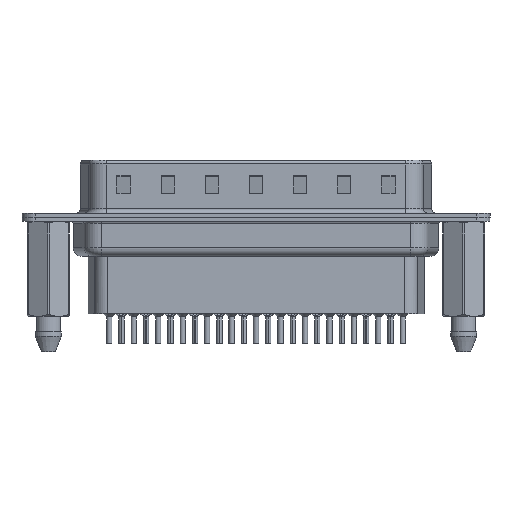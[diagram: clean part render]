
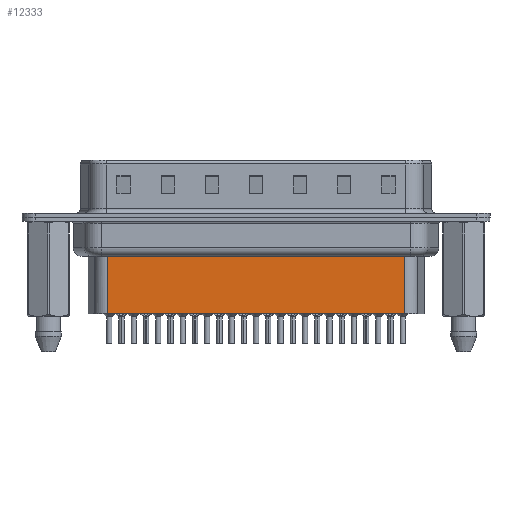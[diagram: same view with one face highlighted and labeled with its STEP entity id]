
A CAD part, front view. The second image highlights one B-rep face of the part: STEP entity #12333.
In plain terms, the highlighted planar face has unit normal (0, -1, 0).
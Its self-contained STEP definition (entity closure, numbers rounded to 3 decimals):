
#512 = VECTOR ( 'NONE', #2384, 1000. ) ;
#756 = CARTESIAN_POINT ( 'NONE',  ( 6.706, -3.5, -3.1 ) ) ;
#787 = FACE_OUTER_BOUND ( 'NONE', #13204, .T. ) ;
#915 = VECTOR ( 'NONE', #7128, 1000. ) ;
#1347 = DIRECTION ( 'NONE',  ( -1., 0., 0. ) ) ;
#1671 = AXIS2_PLACEMENT_3D ( 'NONE', #18731, #20494, #11427 ) ;
#1824 = VERTEX_POINT ( 'NONE', #12395 ) ;
#2384 = DIRECTION ( 'NONE',  ( 0., 0., -1. ) ) ;
#2472 = VERTEX_POINT ( 'NONE', #3318 ) ;
#3318 = CARTESIAN_POINT ( 'NONE',  ( 40.344, -3.5, -10.95 ) ) ;
#4831 = ORIENTED_EDGE ( 'NONE', *, *, #15955, .F. ) ;
#6227 = EDGE_CURVE ( 'NONE', #1824, #2472, #9227, .T. ) ;
#7128 = DIRECTION ( 'NONE',  ( -1., 0., 0. ) ) ;
#7300 = LINE ( 'NONE', #756, #17808 ) ;
#7325 = CARTESIAN_POINT ( 'NONE',  ( 6.706, -3.5, -10.95 ) ) ;
#9227 = LINE ( 'NONE', #20059, #512 ) ;
#9673 = PLANE ( 'NONE',  #1671 ) ;
#11427 = DIRECTION ( 'NONE',  ( 1., 0., 0. ) ) ;
#12333 = ADVANCED_FACE ( 'NONE', ( #787 ), #9673, .T. ) ;
#12395 = CARTESIAN_POINT ( 'NONE',  ( 40.344, -3.5, -4.097 ) ) ;
#12440 = LINE ( 'NONE', #21344, #27753 ) ;
#13204 = EDGE_LOOP ( 'NONE', ( #22185, #24298, #17603, #4831 ) ) ;
#13380 = CARTESIAN_POINT ( 'NONE',  ( 6.706, -3.5, -4.097 ) ) ;
#15955 = EDGE_CURVE ( 'NONE', #2472, #22702, #12440, .T. ) ;
#17603 = ORIENTED_EDGE ( 'NONE', *, *, #24813, .T. ) ;
#17808 = VECTOR ( 'NONE', #25112, 1000. ) ;
#18731 = CARTESIAN_POINT ( 'NONE',  ( 6.706, -3.5, -3.1 ) ) ;
#20059 = CARTESIAN_POINT ( 'NONE',  ( 40.344, -3.5, -3.1 ) ) ;
#20494 = DIRECTION ( 'NONE',  ( 0., -1., 0. ) ) ;
#20744 = CARTESIAN_POINT ( 'NONE',  ( 6.459, -3.5, -4.097 ) ) ;
#21344 = CARTESIAN_POINT ( 'NONE',  ( 6.706, -3.5, -10.95 ) ) ;
#21765 = EDGE_CURVE ( 'NONE', #1824, #28770, #24797, .T. ) ;
#22185 = ORIENTED_EDGE ( 'NONE', *, *, #6227, .F. ) ;
#22702 = VERTEX_POINT ( 'NONE', #7325 ) ;
#24298 = ORIENTED_EDGE ( 'NONE', *, *, #21765, .T. ) ;
#24797 = LINE ( 'NONE', #20744, #915 ) ;
#24813 = EDGE_CURVE ( 'NONE', #28770, #22702, #7300, .T. ) ;
#25112 = DIRECTION ( 'NONE',  ( 0., 0., -1. ) ) ;
#27753 = VECTOR ( 'NONE', #1347, 1000. ) ;
#28770 = VERTEX_POINT ( 'NONE', #13380 ) ;
